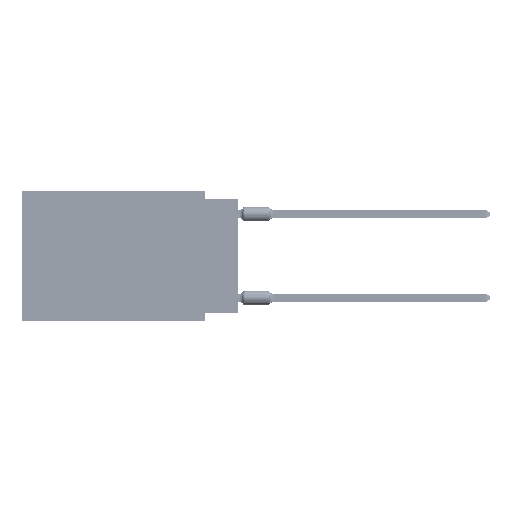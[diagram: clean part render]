
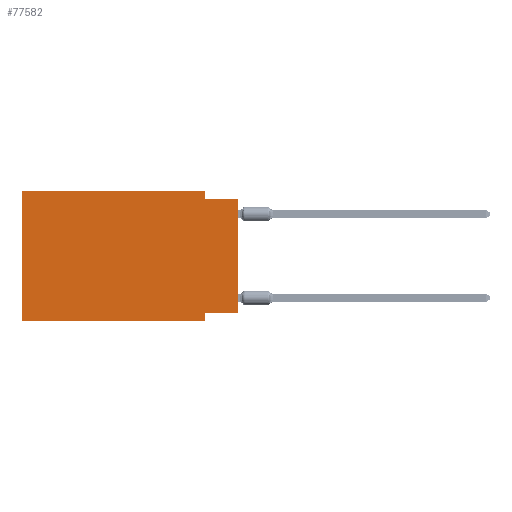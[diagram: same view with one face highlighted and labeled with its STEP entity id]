
A CAD part, left-side view. The second image highlights one B-rep face of the part: STEP entity #77582.
In plain terms, the highlighted planar face has unit normal (-1, 0, 0).
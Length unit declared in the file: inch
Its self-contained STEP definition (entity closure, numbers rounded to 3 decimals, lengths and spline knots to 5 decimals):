
#552 = DIRECTION ( 'NONE',  ( 0., 0., 1. ) ) ;
#2769 = VECTOR ( 'NONE', #11276, 39.37008 ) ;
#2871 = VERTEX_POINT ( 'NONE', #14027 ) ;
#4384 = CARTESIAN_POINT ( 'NONE',  ( 0., 0.1, 0. ) ) ;
#6347 = CARTESIAN_POINT ( 'NONE',  ( 0., 0.1, -0.365 ) ) ;
#11276 = DIRECTION ( 'NONE',  ( 0., 1., 0. ) ) ;
#11650 = FACE_OUTER_BOUND ( 'NONE', #74685, .T. ) ;
#12417 = EDGE_CURVE ( 'NONE', #38042, #78215, #77609, .T. ) ;
#12559 = DIRECTION ( 'NONE',  ( 0., 0., -1. ) ) ;
#13324 = ORIENTED_EDGE ( 'NONE', *, *, #86919, .T. ) ;
#13371 = EDGE_CURVE ( 'NONE', #16299, #63456, #71031, .T. ) ;
#13739 = LINE ( 'NONE', #55251, #14803 ) ;
#14027 = CARTESIAN_POINT ( 'NONE',  ( 0., 0., -0.365 ) ) ;
#14803 = VECTOR ( 'NONE', #552, 39.37008 ) ;
#15168 = DIRECTION ( 'NONE',  ( 0., -1., 0. ) ) ;
#16299 = VERTEX_POINT ( 'NONE', #6347 ) ;
#18166 = ORIENTED_EDGE ( 'NONE', *, *, #12417, .F. ) ;
#18568 = ORIENTED_EDGE ( 'NONE', *, *, #27307, .T. ) ;
#18904 = CARTESIAN_POINT ( 'NONE',  ( 0., 0.645, 0. ) ) ;
#19403 = DIRECTION ( 'NONE',  ( 1., 0., 0. ) ) ;
#23436 = CARTESIAN_POINT ( 'NONE',  ( 0., 0., 0. ) ) ;
#25988 = CARTESIAN_POINT ( 'NONE',  ( 0., 0.1, -0.39 ) ) ;
#27307 = EDGE_CURVE ( 'NONE', #2871, #78215, #85434, .T. ) ;
#28337 = ORIENTED_EDGE ( 'NONE', *, *, #28426, .F. ) ;
#28426 = EDGE_CURVE ( 'NONE', #71891, #51953, #13739, .T. ) ;
#28645 = ORIENTED_EDGE ( 'NONE', *, *, #58056, .F. ) ;
#28929 = VECTOR ( 'NONE', #57164, 39.37008 ) ;
#31722 = VECTOR ( 'NONE', #60426, 39.37008 ) ;
#31802 = VECTOR ( 'NONE', #15168, 39.37008 ) ;
#35044 = VECTOR ( 'NONE', #42627, 39.37008 ) ;
#36383 = CARTESIAN_POINT ( 'NONE',  ( 0., 0.1, -0.39 ) ) ;
#37547 = EDGE_CURVE ( 'NONE', #2871, #16299, #74625, .T. ) ;
#38042 = VERTEX_POINT ( 'NONE', #61299 ) ;
#42627 = DIRECTION ( 'NONE',  ( 0., 0., 1. ) ) ;
#44777 = CARTESIAN_POINT ( 'NONE',  ( 0., 0., -0.025 ) ) ;
#45873 = LINE ( 'NONE', #4384, #31722 ) ;
#47175 = LINE ( 'NONE', #18904, #83405 ) ;
#49890 = CARTESIAN_POINT ( 'NONE',  ( 0., 0.645, -0.39 ) ) ;
#51953 = VERTEX_POINT ( 'NONE', #72685 ) ;
#52812 = VERTEX_POINT ( 'NONE', #85580 ) ;
#54507 = PLANE ( 'NONE',  #57080 ) ;
#55251 = CARTESIAN_POINT ( 'NONE',  ( 0., 0.645, 0. ) ) ;
#55365 = DIRECTION ( 'NONE',  ( 0., -1., 0. ) ) ;
#57080 = AXIS2_PLACEMENT_3D ( 'NONE', #60429, #19403, #12559 ) ;
#57164 = DIRECTION ( 'NONE',  ( 0., -1., 0. ) ) ;
#58056 = EDGE_CURVE ( 'NONE', #51953, #52812, #47175, .T. ) ;
#60426 = DIRECTION ( 'NONE',  ( 0., 0., -1. ) ) ;
#60429 = CARTESIAN_POINT ( 'NONE',  ( 0., 0.645, 0. ) ) ;
#60566 = ORIENTED_EDGE ( 'NONE', *, *, #37547, .F. ) ;
#61299 = CARTESIAN_POINT ( 'NONE',  ( 0., 0.1, -0.025 ) ) ;
#62606 = CARTESIAN_POINT ( 'NONE',  ( 0., 0., -0.025 ) ) ;
#62916 = CARTESIAN_POINT ( 'NONE',  ( 0., 0.645, -0.39 ) ) ;
#63456 = VERTEX_POINT ( 'NONE', #25988 ) ;
#65528 = DIRECTION ( 'NONE',  ( 0., 0., -1. ) ) ;
#70380 = LINE ( 'NONE', #49890, #28929 ) ;
#71031 = LINE ( 'NONE', #36383, #76807 ) ;
#71891 = VERTEX_POINT ( 'NONE', #62916 ) ;
#72685 = CARTESIAN_POINT ( 'NONE',  ( 0., 0.645, 0. ) ) ;
#74625 = LINE ( 'NONE', #88287, #2769 ) ;
#74685 = EDGE_LOOP ( 'NONE', ( #18568, #18166, #74812, #28645, #28337, #13324, #85571, #60566 ) ) ;
#74812 = ORIENTED_EDGE ( 'NONE', *, *, #85894, .F. ) ;
#76807 = VECTOR ( 'NONE', #65528, 39.37008 ) ;
#77582 = ADVANCED_FACE ( 'NONE', ( #11650 ), #54507, .F. ) ;
#77609 = LINE ( 'NONE', #62606, #31802 ) ;
#78215 = VERTEX_POINT ( 'NONE', #44777 ) ;
#83405 = VECTOR ( 'NONE', #55365, 39.37008 ) ;
#85434 = LINE ( 'NONE', #23436, #35044 ) ;
#85571 = ORIENTED_EDGE ( 'NONE', *, *, #13371, .F. ) ;
#85580 = CARTESIAN_POINT ( 'NONE',  ( 0., 0.1, 0. ) ) ;
#85894 = EDGE_CURVE ( 'NONE', #52812, #38042, #45873, .T. ) ;
#86919 = EDGE_CURVE ( 'NONE', #71891, #63456, #70380, .T. ) ;
#88287 = CARTESIAN_POINT ( 'NONE',  ( 0., 0., -0.365 ) ) ;
